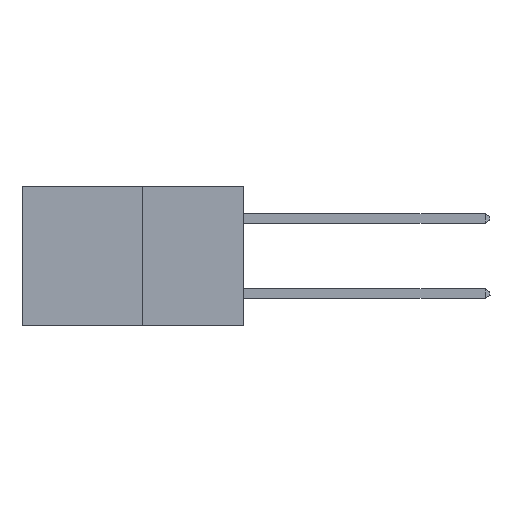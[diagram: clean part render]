
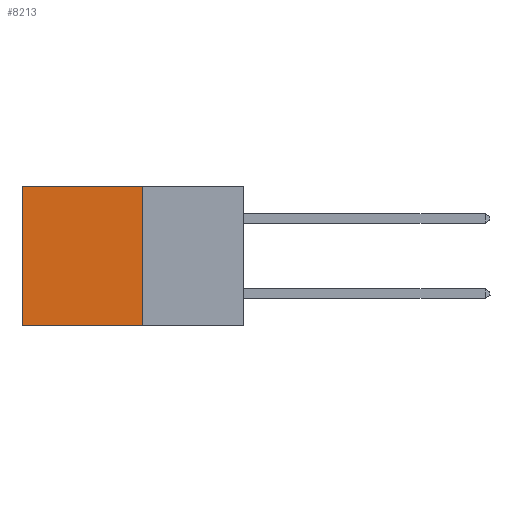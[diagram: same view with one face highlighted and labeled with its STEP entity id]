
A CAD part, left-side view. The second image highlights one B-rep face of the part: STEP entity #8213.
In plain terms, the highlighted planar face has unit normal (-1, 0, 0).
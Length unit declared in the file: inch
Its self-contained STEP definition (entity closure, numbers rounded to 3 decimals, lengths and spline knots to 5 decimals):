
#1725 = ORIENTED_EDGE ( 'NONE', *, *, #22843, .T. ) ;
#1953 = DIRECTION ( 'NONE',  ( 0., 1., 0. ) ) ;
#2199 = CARTESIAN_POINT ( 'NONE',  ( 0.277, 0.27, -0.37 ) ) ;
#4637 = DIRECTION ( 'NONE',  ( 0., 0., -1. ) ) ;
#5518 = VECTOR ( 'NONE', #17078, 39.37008 ) ;
#6787 = PLANE ( 'NONE',  #26872 ) ;
#6927 = EDGE_LOOP ( 'NONE', ( #1725, #20609, #16432, #11289 ) ) ;
#8213 = ADVANCED_FACE ( 'NONE', ( #28619 ), #6787, .F. ) ;
#8791 = VECTOR ( 'NONE', #18572, 39.37008 ) ;
#9795 = CARTESIAN_POINT ( 'NONE',  ( 0.277, 0.27, 0. ) ) ;
#9887 = VERTEX_POINT ( 'NONE', #14770 ) ;
#11289 = ORIENTED_EDGE ( 'NONE', *, *, #14520, .T. ) ;
#11945 = VECTOR ( 'NONE', #1953, 39.37008 ) ;
#12709 = LINE ( 'NONE', #21664, #11945 ) ;
#13534 = EDGE_CURVE ( 'NONE', #19976, #22776, #12709, .T. ) ;
#14520 = EDGE_CURVE ( 'NONE', #19434, #9887, #21772, .T. ) ;
#14770 = CARTESIAN_POINT ( 'NONE',  ( 0.277, 0.59, 0. ) ) ;
#16071 = CARTESIAN_POINT ( 'NONE',  ( 0.277, 0.27, 0. ) ) ;
#16432 = ORIENTED_EDGE ( 'NONE', *, *, #27557, .F. ) ;
#16866 = CARTESIAN_POINT ( 'NONE',  ( 0.277, 0.59, -0.37 ) ) ;
#17078 = DIRECTION ( 'NONE',  ( 0., 0., -1. ) ) ;
#18536 = VECTOR ( 'NONE', #4637, 39.37008 ) ;
#18572 = DIRECTION ( 'NONE',  ( 0., 1., 0. ) ) ;
#19434 = VERTEX_POINT ( 'NONE', #9795 ) ;
#19847 = CARTESIAN_POINT ( 'NONE',  ( 0.277, 0.27, -0.37 ) ) ;
#19955 = DIRECTION ( 'NONE',  ( 0., 0., -1. ) ) ;
#19976 = VERTEX_POINT ( 'NONE', #2199 ) ;
#20609 = ORIENTED_EDGE ( 'NONE', *, *, #13534, .F. ) ;
#21664 = CARTESIAN_POINT ( 'NONE',  ( 0.277, 0.27, -0.37 ) ) ;
#21772 = LINE ( 'NONE', #16071, #8791 ) ;
#22776 = VERTEX_POINT ( 'NONE', #16866 ) ;
#22843 = EDGE_CURVE ( 'NONE', #9887, #22776, #24227, .T. ) ;
#24227 = LINE ( 'NONE', #29074, #5518 ) ;
#24914 = LINE ( 'NONE', #26513, #18536 ) ;
#25294 = DIRECTION ( 'NONE',  ( 1., 0., 0. ) ) ;
#26513 = CARTESIAN_POINT ( 'NONE',  ( 0.277, 0.27, -0.37 ) ) ;
#26872 = AXIS2_PLACEMENT_3D ( 'NONE', #19847, #25294, #19955 ) ;
#27557 = EDGE_CURVE ( 'NONE', #19434, #19976, #24914, .T. ) ;
#28619 = FACE_OUTER_BOUND ( 'NONE', #6927, .T. ) ;
#29074 = CARTESIAN_POINT ( 'NONE',  ( 0.277, 0.59, -0.37 ) ) ;
